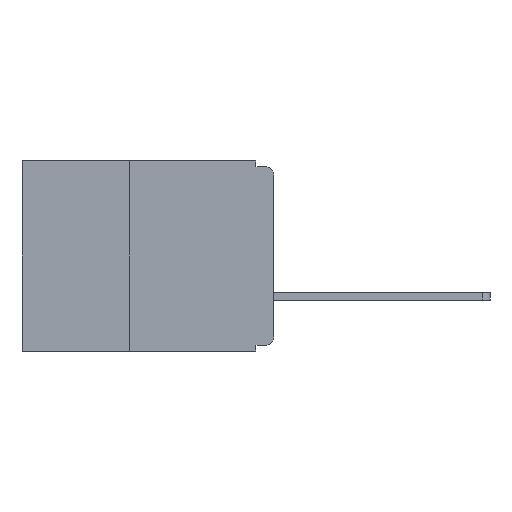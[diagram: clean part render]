
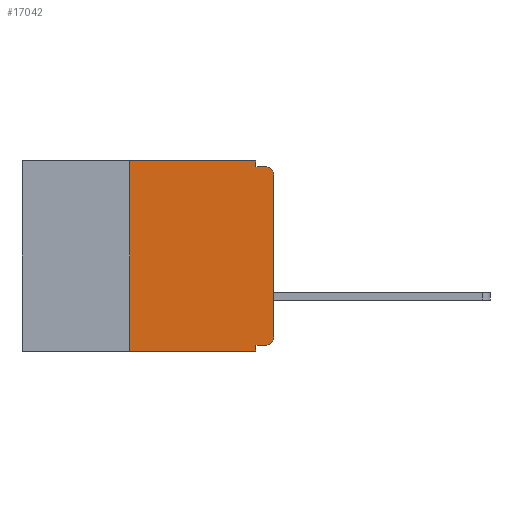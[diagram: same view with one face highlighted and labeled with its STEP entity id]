
A CAD part, left-side view. The second image highlights one B-rep face of the part: STEP entity #17042.
In plain terms, the highlighted planar face has unit normal (-1, 0, 0).
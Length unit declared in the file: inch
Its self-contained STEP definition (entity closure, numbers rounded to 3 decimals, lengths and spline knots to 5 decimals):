
#530 = VECTOR ( 'NONE', #3910, 39.37008 ) ;
#608 = VERTEX_POINT ( 'NONE', #7192 ) ;
#999 = ORIENTED_EDGE ( 'NONE', *, *, #5011, .F. ) ;
#1245 = CARTESIAN_POINT ( 'NONE',  ( 0., 0.031, -0.33 ) ) ;
#1612 = CARTESIAN_POINT ( 'NONE',  ( 0., 0.015, -0.32 ) ) ;
#1764 = CARTESIAN_POINT ( 'NONE',  ( 0., 0., 0. ) ) ;
#2060 = VECTOR ( 'NONE', #7955, 39.37008 ) ;
#3435 = CARTESIAN_POINT ( 'NONE',  ( 0., 0.015, -0.025 ) ) ;
#3910 = DIRECTION ( 'NONE',  ( 0., 0., -1. ) ) ;
#4709 = CARTESIAN_POINT ( 'NONE',  ( 0., 0.015, -0.305 ) ) ;
#4825 = CARTESIAN_POINT ( 'NONE',  ( 0., 0.25, -0.33 ) ) ;
#4965 = AXIS2_PLACEMENT_3D ( 'NONE', #4709, #22965, #7397 ) ;
#5011 = EDGE_CURVE ( 'NONE', #5382, #29190, #5303, .T. ) ;
#5303 = LINE ( 'NONE', #27026, #19999 ) ;
#5382 = VERTEX_POINT ( 'NONE', #12907 ) ;
#5578 = VECTOR ( 'NONE', #25988, 39.37008 ) ;
#6155 = DIRECTION ( 'NONE',  ( 0., 0., -1. ) ) ;
#6338 = VERTEX_POINT ( 'NONE', #24341 ) ;
#6372 = CARTESIAN_POINT ( 'NONE',  ( 0., 0.031, 0. ) ) ;
#6859 = ORIENTED_EDGE ( 'NONE', *, *, #11454, .F. ) ;
#7192 = CARTESIAN_POINT ( 'NONE',  ( 0., 0., -0.305 ) ) ;
#7355 = PLANE ( 'NONE',  #18563 ) ;
#7397 = DIRECTION ( 'NONE',  ( 0., 0., -1. ) ) ;
#7955 = DIRECTION ( 'NONE',  ( 0., -1., 0. ) ) ;
#8577 = DIRECTION ( 'NONE',  ( 0., -1., 0. ) ) ;
#9202 = CARTESIAN_POINT ( 'NONE',  ( 0., 0.031, -0.33 ) ) ;
#9534 = CARTESIAN_POINT ( 'NONE',  ( 0., 0.031, -0.01 ) ) ;
#9575 = VERTEX_POINT ( 'NONE', #9202 ) ;
#9960 = DIRECTION ( 'NONE',  ( 0., 0., -1. ) ) ;
#10389 = CARTESIAN_POINT ( 'NONE',  ( 0., 0.25, -0.33 ) ) ;
#11206 = CIRCLE ( 'NONE', #4965, 0.015 ) ;
#11239 = ORIENTED_EDGE ( 'NONE', *, *, #26528, .F. ) ;
#11423 = DIRECTION ( 'NONE',  ( 0., -1., 0. ) ) ;
#11454 = EDGE_CURVE ( 'NONE', #29190, #11620, #32921, .T. ) ;
#11620 = VERTEX_POINT ( 'NONE', #9534 ) ;
#11707 = ORIENTED_EDGE ( 'NONE', *, *, #21053, .F. ) ;
#12319 = LINE ( 'NONE', #1764, #24533 ) ;
#12522 = LINE ( 'NONE', #10389, #5578 ) ;
#12677 = EDGE_CURVE ( 'NONE', #21657, #6338, #23872, .T. ) ;
#12907 = CARTESIAN_POINT ( 'NONE',  ( 0., 0.25, 0. ) ) ;
#13484 = EDGE_CURVE ( 'NONE', #15178, #608, #11206, .T. ) ;
#13610 = VERTEX_POINT ( 'NONE', #20792 ) ;
#13999 = CARTESIAN_POINT ( 'NONE',  ( 0., 0.031, 0. ) ) ;
#15178 = VERTEX_POINT ( 'NONE', #1612 ) ;
#15189 = ORIENTED_EDGE ( 'NONE', *, *, #33768, .F. ) ;
#15684 = AXIS2_PLACEMENT_3D ( 'NONE', #3435, #21745, #6155 ) ;
#15943 = ORIENTED_EDGE ( 'NONE', *, *, #19756, .T. ) ;
#16605 = DIRECTION ( 'NONE',  ( 0., 0., -1. ) ) ;
#17042 = ADVANCED_FACE ( 'NONE', ( #28801 ), #7355, .F. ) ;
#17665 = VECTOR ( 'NONE', #30175, 39.37008 ) ;
#17708 = CARTESIAN_POINT ( 'NONE',  ( 0., 0.437, 0. ) ) ;
#18563 = AXIS2_PLACEMENT_3D ( 'NONE', #17708, #25547, #9960 ) ;
#19756 = EDGE_CURVE ( 'NONE', #608, #21657, #12319, .T. ) ;
#19823 = VERTEX_POINT ( 'NONE', #4825 ) ;
#19999 = VECTOR ( 'NONE', #11423, 39.37008 ) ;
#20342 = ORIENTED_EDGE ( 'NONE', *, *, #13484, .T. ) ;
#20792 = CARTESIAN_POINT ( 'NONE',  ( 0., 0.031, -0.32 ) ) ;
#21053 = EDGE_CURVE ( 'NONE', #11620, #6338, #24903, .T. ) ;
#21471 = LINE ( 'NONE', #1245, #530 ) ;
#21657 = VERTEX_POINT ( 'NONE', #24656 ) ;
#21745 = DIRECTION ( 'NONE',  ( -1., 0., 0. ) ) ;
#22853 = DIRECTION ( 'NONE',  ( 0., 0., 1. ) ) ;
#22965 = DIRECTION ( 'NONE',  ( -1., 0., 0. ) ) ;
#23395 = EDGE_CURVE ( 'NONE', #13610, #9575, #21471, .T. ) ;
#23789 = LINE ( 'NONE', #33763, #2060 ) ;
#23872 = CIRCLE ( 'NONE', #15684, 0.015 ) ;
#24133 = CARTESIAN_POINT ( 'NONE',  ( 0., 0., -0.01 ) ) ;
#24341 = CARTESIAN_POINT ( 'NONE',  ( 0., 0.015, -0.01 ) ) ;
#24533 = VECTOR ( 'NONE', #22853, 39.37008 ) ;
#24574 = LINE ( 'NONE', #24968, #17665 ) ;
#24656 = CARTESIAN_POINT ( 'NONE',  ( 0., 0., -0.025 ) ) ;
#24903 = LINE ( 'NONE', #24133, #25718 ) ;
#24968 = CARTESIAN_POINT ( 'NONE',  ( 0., 0., -0.32 ) ) ;
#25547 = DIRECTION ( 'NONE',  ( 1., 0., 0. ) ) ;
#25718 = VECTOR ( 'NONE', #8577, 39.37008 ) ;
#25988 = DIRECTION ( 'NONE',  ( 0., 0., 1. ) ) ;
#26182 = EDGE_CURVE ( 'NONE', #19823, #9575, #23789, .T. ) ;
#26528 = EDGE_CURVE ( 'NONE', #15178, #13610, #24574, .T. ) ;
#27026 = CARTESIAN_POINT ( 'NONE',  ( 0., 0.437, 0. ) ) ;
#27598 = VECTOR ( 'NONE', #16605, 39.37008 ) ;
#28550 = EDGE_LOOP ( 'NONE', ( #15943, #31510, #11707, #6859, #999, #15189, #32721, #33207, #11239, #20342 ) ) ;
#28801 = FACE_OUTER_BOUND ( 'NONE', #28550, .T. ) ;
#29190 = VERTEX_POINT ( 'NONE', #6372 ) ;
#30175 = DIRECTION ( 'NONE',  ( 0., 1., 0. ) ) ;
#31510 = ORIENTED_EDGE ( 'NONE', *, *, #12677, .T. ) ;
#32721 = ORIENTED_EDGE ( 'NONE', *, *, #26182, .T. ) ;
#32921 = LINE ( 'NONE', #13999, #27598 ) ;
#33207 = ORIENTED_EDGE ( 'NONE', *, *, #23395, .F. ) ;
#33763 = CARTESIAN_POINT ( 'NONE',  ( 0., 0.437, -0.33 ) ) ;
#33768 = EDGE_CURVE ( 'NONE', #19823, #5382, #12522, .T. ) ;
